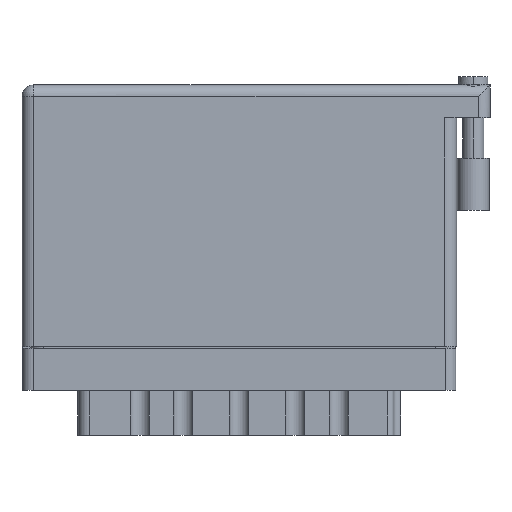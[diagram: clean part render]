
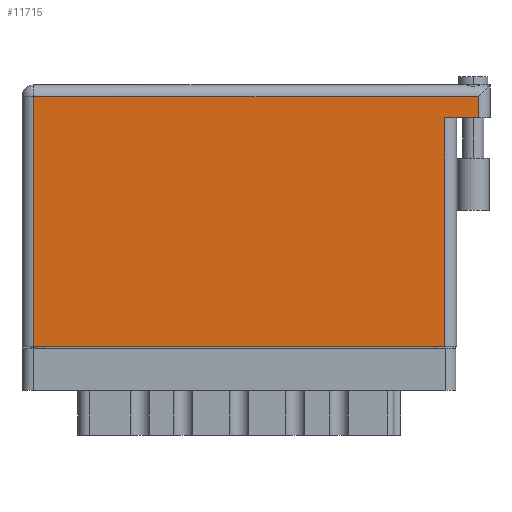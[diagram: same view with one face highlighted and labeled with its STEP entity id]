
A CAD part, front view. The second image highlights one B-rep face of the part: STEP entity #11715.
In plain terms, the highlighted face is planar.
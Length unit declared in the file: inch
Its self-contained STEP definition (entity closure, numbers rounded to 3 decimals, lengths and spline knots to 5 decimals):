
#69 = VECTOR ( 'NONE', #37220, 39.37008 ) ;
#3089 = EDGE_CURVE ( 'NONE', #49120, #40743, #8940, .T. ) ;
#5219 = CARTESIAN_POINT ( 'NONE',  ( 2.73, 1.369, 0. ) ) ;
#6034 = VECTOR ( 'NONE', #45557, 39.37008 ) ;
#6177 = EDGE_CURVE ( 'NONE', #25776, #22387, #29528, .T. ) ;
#6399 = CARTESIAN_POINT ( 'NONE',  ( 2.53, 1.369, 0. ) ) ;
#8940 = LINE ( 'NONE', #43998, #69 ) ;
#9184 = VECTOR ( 'NONE', #22988, 39.37008 ) ;
#10097 = LINE ( 'NONE', #6399, #37521 ) ;
#10552 = DIRECTION ( 'NONE',  ( -1., 0., 0. ) ) ;
#11715 = ADVANCED_FACE ( 'NONE', ( #25720 ), #14370, .F. ) ;
#12425 = VECTOR ( 'NONE', #10552, 39.37008 ) ;
#12544 = EDGE_CURVE ( 'NONE', #22387, #14862, #32790, .T. ) ;
#14370 = PLANE ( 'NONE',  #17993 ) ;
#14862 = VERTEX_POINT ( 'NONE', #25471 ) ;
#16299 = EDGE_LOOP ( 'NONE', ( #21781, #45403, #38581, #22280, #20285, #37145 ) ) ;
#17747 = CARTESIAN_POINT ( 'NONE',  ( 0.07, 0., 0. ) ) ;
#17993 = AXIS2_PLACEMENT_3D ( 'NONE', #32503, #22765, #31293 ) ;
#18064 = EDGE_CURVE ( 'NONE', #14862, #49120, #32423, .T. ) ;
#20285 = ORIENTED_EDGE ( 'NONE', *, *, #12544, .T. ) ;
#21781 = ORIENTED_EDGE ( 'NONE', *, *, #3089, .T. ) ;
#22280 = ORIENTED_EDGE ( 'NONE', *, *, #6177, .T. ) ;
#22387 = VERTEX_POINT ( 'NONE', #39943 ) ;
#22765 = DIRECTION ( 'NONE',  ( 0., 0., -1. ) ) ;
#22988 = DIRECTION ( 'NONE',  ( 0., -1., 0. ) ) ;
#23547 = EDGE_CURVE ( 'NONE', #40743, #40654, #10097, .T. ) ;
#23772 = EDGE_CURVE ( 'NONE', #25776, #40654, #30277, .T. ) ;
#25471 = CARTESIAN_POINT ( 'NONE',  ( 0.07, 1.496, 0. ) ) ;
#25720 = FACE_OUTER_BOUND ( 'NONE', #16299, .T. ) ;
#25776 = VERTEX_POINT ( 'NONE', #5219 ) ;
#29528 = LINE ( 'NONE', #43946, #33112 ) ;
#29647 = CARTESIAN_POINT ( 'NONE',  ( 2.53, 1.369, 0. ) ) ;
#30256 = CARTESIAN_POINT ( 'NONE',  ( 0., 1.496, 0. ) ) ;
#30277 = LINE ( 'NONE', #41490, #12425 ) ;
#31293 = DIRECTION ( 'NONE',  ( -1., 0., 0. ) ) ;
#32423 = LINE ( 'NONE', #38667, #9184 ) ;
#32503 = CARTESIAN_POINT ( 'NONE',  ( 0., 1.566, 0. ) ) ;
#32790 = LINE ( 'NONE', #30256, #6034 ) ;
#33112 = VECTOR ( 'NONE', #36481, 39.37008 ) ;
#36481 = DIRECTION ( 'NONE',  ( 0., 1., 0. ) ) ;
#37145 = ORIENTED_EDGE ( 'NONE', *, *, #18064, .T. ) ;
#37220 = DIRECTION ( 'NONE',  ( 1., 0., 0. ) ) ;
#37521 = VECTOR ( 'NONE', #48122, 39.37008 ) ;
#38581 = ORIENTED_EDGE ( 'NONE', *, *, #23772, .F. ) ;
#38667 = CARTESIAN_POINT ( 'NONE',  ( 0.07, 0., 0. ) ) ;
#39943 = CARTESIAN_POINT ( 'NONE',  ( 2.73, 1.496, 0. ) ) ;
#40654 = VERTEX_POINT ( 'NONE', #29647 ) ;
#40743 = VERTEX_POINT ( 'NONE', #45570 ) ;
#41490 = CARTESIAN_POINT ( 'NONE',  ( 2.8, 1.369, 0. ) ) ;
#43946 = CARTESIAN_POINT ( 'NONE',  ( 2.73, 1.566, 0. ) ) ;
#43998 = CARTESIAN_POINT ( 'NONE',  ( 0., 0., 0. ) ) ;
#45403 = ORIENTED_EDGE ( 'NONE', *, *, #23547, .T. ) ;
#45557 = DIRECTION ( 'NONE',  ( -1., 0., 0. ) ) ;
#45570 = CARTESIAN_POINT ( 'NONE',  ( 2.53, 0., 0. ) ) ;
#48122 = DIRECTION ( 'NONE',  ( 0., 1., 0. ) ) ;
#49120 = VERTEX_POINT ( 'NONE', #17747 ) ;
